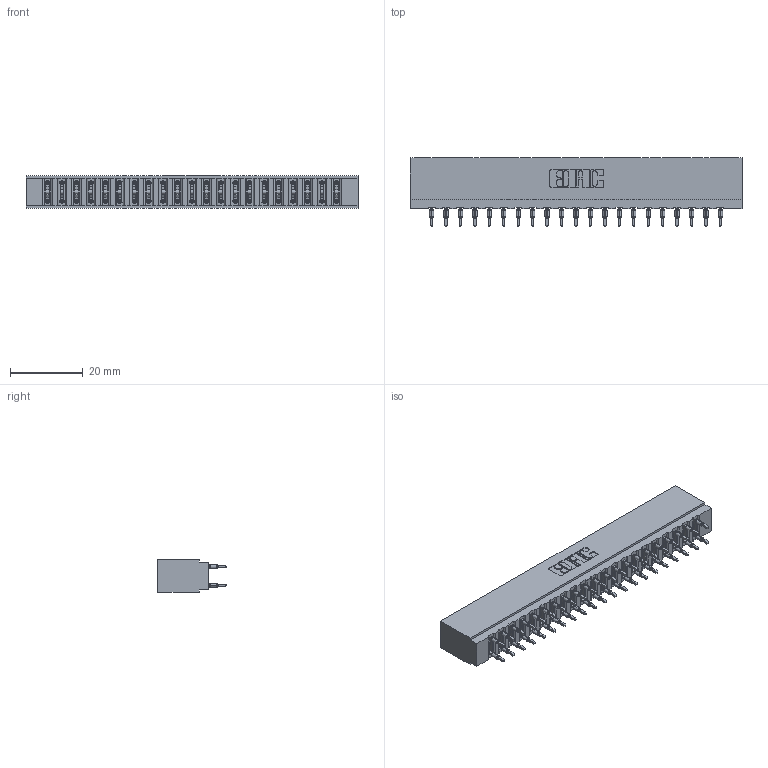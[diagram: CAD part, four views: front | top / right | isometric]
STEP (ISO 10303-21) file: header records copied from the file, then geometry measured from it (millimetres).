
FILE_DESCRIPTION (( 'STEP AP203' ), '1' );
FILE_NAME ('717-042-560-201.STEP', '2026-02-20T17:59:04', ( '' ), ( '' ), 'SwSTEP 2.0', 'SolidWorks 2023', '' );
FILE_SCHEMA (( 'CONFIG_CONTROL_DESIGN' ));
Length unit declared in the file: millimetre
Products named in the file (3): 717 Part_Insulator Option - 06; 717-042-560-201; 745-292-001_560
Assembly tree (43 placements, depth 2):
  717-042-560-201
    717 Part_Insulator Option - 06
    745-292-001_560  x42
Bounding box: 91.08 x 18.78 x 8.89 mm (x, y, z)
Volume: 8134.5 mm3; surface area: 12900.7 mm2
Topology: 43 solids, 43 shells, 4252 faces, 11633 edges, 7390 vertices
Faces by surface type: plane 2217, cylinder 943, bspline 840, torus 252
Entity records: 39168 total; most frequent: CARTESIAN_POINT 7309, ORIENTED_EDGE 6702, DIRECTION 5875, EDGE_CURVE 3351, LINE 3035, VECTOR 3035, VERTEX_POINT 2142, AXIS2_PLACEMENT_3D 1420
